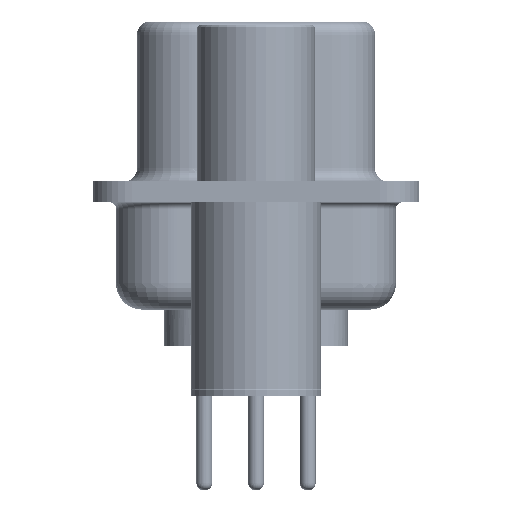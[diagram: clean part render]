
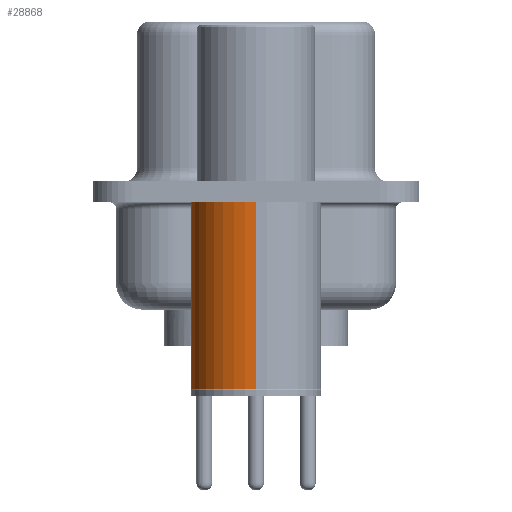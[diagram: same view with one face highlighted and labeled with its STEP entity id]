
A CAD part, left-side view. The second image highlights one B-rep face of the part: STEP entity #28868.
In plain terms, the highlighted cylindrical face has radius 2.5 mm (diameter 5 mm), a partial arc.
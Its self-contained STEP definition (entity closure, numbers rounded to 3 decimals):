
#729 = CYLINDRICAL_SURFACE ( 'NONE', #31652, 2.5 ) ;
#938 = DIRECTION ( 'NONE',  ( 1., 0., 0. ) ) ;
#2768 = EDGE_CURVE ( 'NONE', #6626, #21794, #6995, .T. ) ;
#3462 = EDGE_CURVE ( 'NONE', #6626, #29062, #28535, .T. ) ;
#3657 = DIRECTION ( 'NONE',  ( 0., 0., 1. ) ) ;
#5113 = CARTESIAN_POINT ( 'NONE',  ( 2.5, 0., 0.581 ) ) ;
#5550 = VECTOR ( 'NONE', #16944, 1000. ) ;
#6417 = LINE ( 'NONE', #27384, #5550 ) ;
#6520 = CARTESIAN_POINT ( 'NONE',  ( 0., 0., -0.4 ) ) ;
#6626 = VERTEX_POINT ( 'NONE', #9847 ) ;
#6995 = LINE ( 'NONE', #5113, #34348 ) ;
#7181 = ORIENTED_EDGE ( 'NONE', *, *, #19610, .F. ) ;
#8193 = AXIS2_PLACEMENT_3D ( 'NONE', #13411, #13206, #13077 ) ;
#8930 = AXIS2_PLACEMENT_3D ( 'NONE', #6520, #25073, #9163 ) ;
#9163 = DIRECTION ( 'NONE',  ( 1., 0., 0. ) ) ;
#9847 = CARTESIAN_POINT ( 'NONE',  ( 2.5, 0., -7.525 ) ) ;
#12410 = EDGE_CURVE ( 'NONE', #29062, #15836, #6417, .T. ) ;
#13077 = DIRECTION ( 'NONE',  ( 1., 0., 0. ) ) ;
#13206 = DIRECTION ( 'NONE',  ( 0., 0., 1. ) ) ;
#13411 = CARTESIAN_POINT ( 'NONE',  ( 0., 0., -7.525 ) ) ;
#14225 = EDGE_LOOP ( 'NONE', ( #25525, #26176, #7181, #17539 ) ) ;
#15836 = VERTEX_POINT ( 'NONE', #30775 ) ;
#16944 = DIRECTION ( 'NONE',  ( 0., 0., 1. ) ) ;
#17539 = ORIENTED_EDGE ( 'NONE', *, *, #2768, .F. ) ;
#19610 = EDGE_CURVE ( 'NONE', #21794, #15836, #19846, .T. ) ;
#19683 = CARTESIAN_POINT ( 'NONE',  ( 0., 0., 0.581 ) ) ;
#19846 = CIRCLE ( 'NONE', #8930, 2.5 ) ;
#20336 = DIRECTION ( 'NONE',  ( 0., 0., 1. ) ) ;
#21794 = VERTEX_POINT ( 'NONE', #32043 ) ;
#22026 = FACE_OUTER_BOUND ( 'NONE', #14225, .T. ) ;
#25073 = DIRECTION ( 'NONE',  ( 0., 0., 1. ) ) ;
#25525 = ORIENTED_EDGE ( 'NONE', *, *, #3462, .T. ) ;
#26176 = ORIENTED_EDGE ( 'NONE', *, *, #12410, .T. ) ;
#27384 = CARTESIAN_POINT ( 'NONE',  ( -2.5, 0., 0.581 ) ) ;
#28535 = CIRCLE ( 'NONE', #8193, 2.5 ) ;
#28694 = CARTESIAN_POINT ( 'NONE',  ( -2.5, 0., -7.525 ) ) ;
#28868 = ADVANCED_FACE ( 'NONE', ( #22026 ), #729, .T. ) ;
#29062 = VERTEX_POINT ( 'NONE', #28694 ) ;
#30775 = CARTESIAN_POINT ( 'NONE',  ( -2.5, 0., -0.4 ) ) ;
#31652 = AXIS2_PLACEMENT_3D ( 'NONE', #19683, #3657, #938 ) ;
#32043 = CARTESIAN_POINT ( 'NONE',  ( 2.5, 0., -0.4 ) ) ;
#34348 = VECTOR ( 'NONE', #20336, 1000. ) ;
